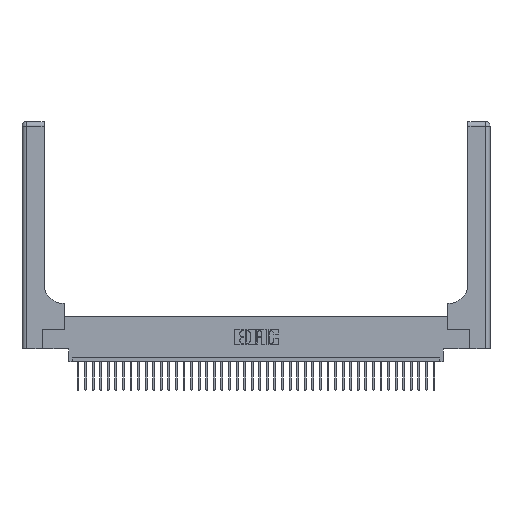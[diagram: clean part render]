
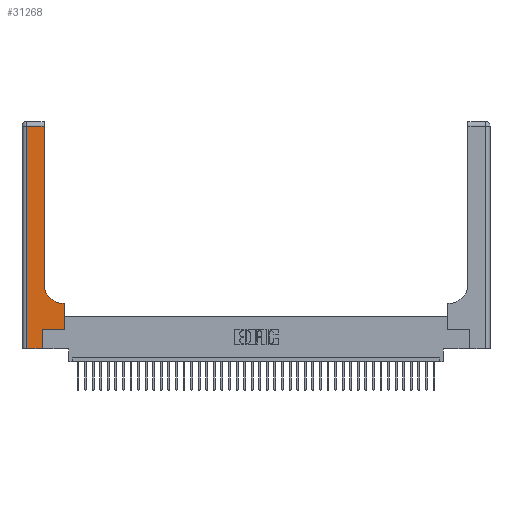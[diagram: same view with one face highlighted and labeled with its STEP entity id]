
A CAD part, top view. The second image highlights one B-rep face of the part: STEP entity #31268.
In plain terms, the highlighted planar face has unit normal (0, 0, 1).
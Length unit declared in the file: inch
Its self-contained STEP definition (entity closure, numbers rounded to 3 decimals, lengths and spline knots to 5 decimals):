
#881 = VECTOR ( 'NONE', #27008, 39.37008 ) ;
#980 = VERTEX_POINT ( 'NONE', #14501 ) ;
#995 = VERTEX_POINT ( 'NONE', #8395 ) ;
#1122 = VERTEX_POINT ( 'NONE', #9122 ) ;
#2268 = CARTESIAN_POINT ( 'NONE',  ( 0.06, 3., 0.37 ) ) ;
#3681 = ORIENTED_EDGE ( 'NONE', *, *, #31146, .T. ) ;
#5071 = VECTOR ( 'NONE', #28099, 39.37008 ) ;
#6377 = EDGE_CURVE ( 'NONE', #40177, #37847, #7595, .T. ) ;
#6541 = ORIENTED_EDGE ( 'NONE', *, *, #25761, .T. ) ;
#6684 = EDGE_CURVE ( 'NONE', #40518, #995, #37058, .T. ) ;
#6796 = LINE ( 'NONE', #11832, #12200 ) ;
#6921 = CARTESIAN_POINT ( 'NONE',  ( 0.06, 0., 0.37 ) ) ;
#7595 = LINE ( 'NONE', #2268, #19322 ) ;
#8395 = CARTESIAN_POINT ( 'NONE',  ( 0.2915, 0.85, 0.37 ) ) ;
#8527 = CARTESIAN_POINT ( 'NONE',  ( 0.5415, 0.6, 0.37 ) ) ;
#9063 = CARTESIAN_POINT ( 'NONE',  ( 0.5415, 0.85, 0.37 ) ) ;
#9065 = CARTESIAN_POINT ( 'NONE',  ( 0.269, 0.25, 0.37 ) ) ;
#9122 = CARTESIAN_POINT ( 'NONE',  ( 0.5585, 0.6, 0.37 ) ) ;
#9582 = VERTEX_POINT ( 'NONE', #17059 ) ;
#11522 = VECTOR ( 'NONE', #27644, 39.37008 ) ;
#11679 = DIRECTION ( 'NONE',  ( -1., 0., 0. ) ) ;
#11832 = CARTESIAN_POINT ( 'NONE',  ( 0.2915, 0.6, 0.37 ) ) ;
#12136 = ORIENTED_EDGE ( 'NONE', *, *, #27748, .T. ) ;
#12200 = VECTOR ( 'NONE', #15244, 39.37008 ) ;
#12633 = ORIENTED_EDGE ( 'NONE', *, *, #6684, .T. ) ;
#12811 = VECTOR ( 'NONE', #29601, 39.37008 ) ;
#13264 = VERTEX_POINT ( 'NONE', #30913 ) ;
#13848 = LINE ( 'NONE', #37445, #14845 ) ;
#14030 = CARTESIAN_POINT ( 'NONE',  ( 0., 3., 0.37 ) ) ;
#14501 = CARTESIAN_POINT ( 'NONE',  ( 0.2915, 2.94, 0.37 ) ) ;
#14845 = VECTOR ( 'NONE', #18598, 39.37008 ) ;
#15244 = DIRECTION ( 'NONE',  ( -1., 0., 0. ) ) ;
#15639 = ORIENTED_EDGE ( 'NONE', *, *, #29336, .T. ) ;
#17059 = CARTESIAN_POINT ( 'NONE',  ( 0.269, 0.25, 0.37 ) ) ;
#18125 = ORIENTED_EDGE ( 'NONE', *, *, #28833, .T. ) ;
#18598 = DIRECTION ( 'NONE',  ( 0., 1., 0. ) ) ;
#18889 = VERTEX_POINT ( 'NONE', #32194 ) ;
#19322 = VECTOR ( 'NONE', #40146, 39.37008 ) ;
#19636 = DIRECTION ( 'NONE',  ( 0., 0., -1. ) ) ;
#19919 = DIRECTION ( 'NONE',  ( -1., 0., 0. ) ) ;
#20222 = LINE ( 'NONE', #22667, #12811 ) ;
#22667 = CARTESIAN_POINT ( 'NONE',  ( 0.2915, 3., 0.37 ) ) ;
#23465 = PLANE ( 'NONE',  #32810 ) ;
#24421 = CARTESIAN_POINT ( 'NONE',  ( 0., 0., 0.37 ) ) ;
#25517 = LINE ( 'NONE', #9065, #5071 ) ;
#25761 = EDGE_CURVE ( 'NONE', #9582, #13264, #25517, .T. ) ;
#25882 = LINE ( 'NONE', #36632, #881 ) ;
#27008 = DIRECTION ( 'NONE',  ( 0., 1., 0. ) ) ;
#27613 = CARTESIAN_POINT ( 'NONE',  ( 0., 2.94, 0.37 ) ) ;
#27644 = DIRECTION ( 'NONE',  ( 1., 0., 0. ) ) ;
#27748 = EDGE_CURVE ( 'NONE', #13264, #1122, #25882, .T. ) ;
#28099 = DIRECTION ( 'NONE',  ( 1., 0., 0. ) ) ;
#28833 = EDGE_CURVE ( 'NONE', #18889, #9582, #13848, .T. ) ;
#29336 = EDGE_CURVE ( 'NONE', #995, #980, #20222, .T. ) ;
#29601 = DIRECTION ( 'NONE',  ( 0., 1., 0. ) ) ;
#30913 = CARTESIAN_POINT ( 'NONE',  ( 0.5585, 0.25, 0.37 ) ) ;
#31146 = EDGE_CURVE ( 'NONE', #1122, #40518, #6796, .T. ) ;
#31268 = ADVANCED_FACE ( 'NONE', ( #33872 ), #23465, .F. ) ;
#32194 = CARTESIAN_POINT ( 'NONE',  ( 0.269, 0., 0.37 ) ) ;
#32244 = DIRECTION ( 'NONE',  ( 1., 0., 0. ) ) ;
#32443 = DIRECTION ( 'NONE',  ( 0., 0., -1. ) ) ;
#32770 = ORIENTED_EDGE ( 'NONE', *, *, #6377, .T. ) ;
#32810 = AXIS2_PLACEMENT_3D ( 'NONE', #14030, #32443, #19919 ) ;
#33156 = ORIENTED_EDGE ( 'NONE', *, *, #39494, .T. ) ;
#33158 = EDGE_CURVE ( 'NONE', #980, #40177, #37621, .T. ) ;
#33872 = FACE_OUTER_BOUND ( 'NONE', #38127, .T. ) ;
#35646 = CARTESIAN_POINT ( 'NONE',  ( 0.06, 2.94, 0.37 ) ) ;
#36599 = LINE ( 'NONE', #24421, #11522 ) ;
#36632 = CARTESIAN_POINT ( 'NONE',  ( 0.5585, 0.25, 0.37 ) ) ;
#37058 = CIRCLE ( 'NONE', #39219, 0.25 ) ;
#37445 = CARTESIAN_POINT ( 'NONE',  ( 0.269, 0., 0.37 ) ) ;
#37621 = LINE ( 'NONE', #27613, #39149 ) ;
#37847 = VERTEX_POINT ( 'NONE', #6921 ) ;
#38127 = EDGE_LOOP ( 'NONE', ( #15639, #40544, #32770, #33156, #18125, #6541, #12136, #3681, #12633 ) ) ;
#39149 = VECTOR ( 'NONE', #11679, 39.37008 ) ;
#39219 = AXIS2_PLACEMENT_3D ( 'NONE', #9063, #19636, #32244 ) ;
#39494 = EDGE_CURVE ( 'NONE', #37847, #18889, #36599, .T. ) ;
#40146 = DIRECTION ( 'NONE',  ( 0., -1., 0. ) ) ;
#40177 = VERTEX_POINT ( 'NONE', #35646 ) ;
#40518 = VERTEX_POINT ( 'NONE', #8527 ) ;
#40544 = ORIENTED_EDGE ( 'NONE', *, *, #33158, .T. ) ;
